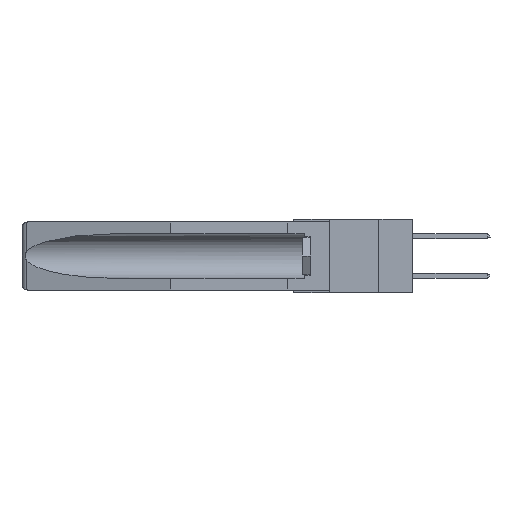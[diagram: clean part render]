
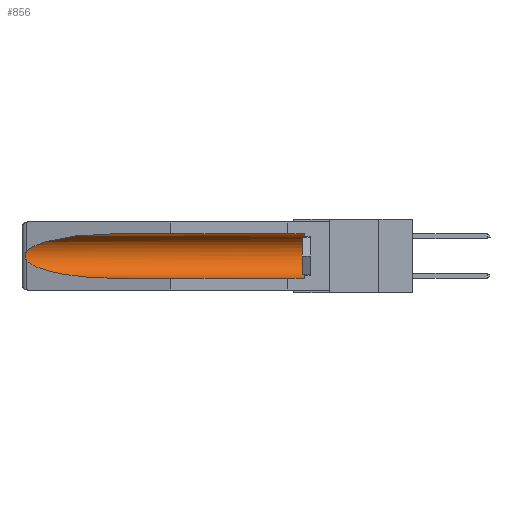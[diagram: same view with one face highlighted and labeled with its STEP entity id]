
A CAD part, left-side view. The second image highlights one B-rep face of the part: STEP entity #856.
In plain terms, the highlighted cylindrical face has radius 2.857 mm (diameter 5.715 mm), a partial arc.
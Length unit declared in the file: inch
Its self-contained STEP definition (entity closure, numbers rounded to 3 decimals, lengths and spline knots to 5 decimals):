
#4 = CARTESIAN_POINT ( 'NONE',  ( 0.26655, 1.53094, -0.18657 ) ) ;
#178 = DIRECTION ( 'NONE',  ( 0., 0., 1. ) ) ;
#856 = ADVANCED_FACE ( 'NONE', ( #16319 ), #3533, .F. ) ;
#969 = VECTOR ( 'NONE', #8975, 39.37008 ) ;
#1082 = ORIENTED_EDGE ( 'NONE', *, *, #8645, .T. ) ;
#1459 = EDGE_CURVE ( 'NONE', #2315, #2692, #11492, .T. ) ;
#2315 = VERTEX_POINT ( 'NONE', #5352 ) ;
#2692 = VERTEX_POINT ( 'NONE', #3282 ) ;
#3206 = ORIENTED_EDGE ( 'NONE', *, *, #9917, .T. ) ;
#3261 = EDGE_CURVE ( 'NONE', #19137, #19927, #17291, .T. ) ;
#3282 = CARTESIAN_POINT ( 'NONE',  ( 0.26537, 1.52718, -0.14972 ) ) ;
#3533 = CYLINDRICAL_SURFACE ( 'NONE', #19335, 0.1125 ) ;
#3579 = VERTEX_POINT ( 'NONE', #5438 ) ;
#3712 = DIRECTION ( 'NONE',  ( 0., 1., 0. ) ) ;
#3803 = CARTESIAN_POINT ( 'NONE',  ( 0.155, 1.07973, -0.284 ) ) ;
#4397 = CARTESIAN_POINT ( 'NONE',  ( 0.26654, 1.53092, -0.15636 ) ) ;
#4469 = EDGE_LOOP ( 'NONE', ( #11773, #3206, #8461, #10026, #18806, #1082 ) ) ;
#5352 = CARTESIAN_POINT ( 'NONE',  ( 0.155, 1.07973, -0.059 ) ) ;
#5438 = CARTESIAN_POINT ( 'NONE',  ( 0.155, 0.126, -0.284 ) ) ;
#5480 = CARTESIAN_POINT ( 'NONE',  ( 0.26537, 1.52718, -0.19328 ) ) ;
#6996 = CARTESIAN_POINT ( 'NONE',  ( 0.25451, 1.48313, -0.24835 ) ) ;
#7425 = CARTESIAN_POINT ( 'NONE',  ( 0.26537, 1.52718, -0.14972 ) ) ;
#7823 = CARTESIAN_POINT ( 'NONE',  ( 0.2675, 1.53308, -0.17534 ) ) ;
#8456 = CARTESIAN_POINT ( 'NONE',  ( 0.21114, 1.30732, -0.059 ) ) ;
#8461 = ORIENTED_EDGE ( 'NONE', *, *, #3261, .T. ) ;
#8645 = EDGE_CURVE ( 'NONE', #19172, #2315, #10836, .T. ) ;
#8659 = CARTESIAN_POINT ( 'NONE',  ( 0.26537, 1.52718, -0.14972 ) ) ;
#8975 = DIRECTION ( 'NONE',  ( 0., 1., 0. ) ) ;
#9210 = EDGE_CURVE ( 'NONE', #3579, #19172, #12037, .T. ) ;
#9917 = EDGE_CURVE ( 'NONE', #2692, #19137, #11753, .T. ) ;
#10026 = ORIENTED_EDGE ( 'NONE', *, *, #10913, .F. ) ;
#10836 = LINE ( 'NONE', #18160, #969 ) ;
#10913 = EDGE_CURVE ( 'NONE', #3579, #19927, #12956, .T. ) ;
#10934 = CARTESIAN_POINT ( 'NONE',  ( 0.26537, 1.52718, -0.19328 ) ) ;
#11492 =( BOUNDED_CURVE ( )  B_SPLINE_CURVE ( 3, ( #11708, #8456, #14905, #8659 ),
 .UNSPECIFIED., .F., .F. ) 
 B_SPLINE_CURVE_WITH_KNOTS ( ( 4, 4 ),
 ( 4.71239, 6.08839 ),
 .UNSPECIFIED. ) 
 CURVE ( )  GEOMETRIC_REPRESENTATION_ITEM ( )  RATIONAL_B_SPLINE_CURVE ( ( 1., 0.848, 0.848, 1. ) ) 
 REPRESENTATION_ITEM ( '' )  );
#11635 = CARTESIAN_POINT ( 'NONE',  ( 0.155, -0.30754, -0.1715 ) ) ;
#11708 = CARTESIAN_POINT ( 'NONE',  ( 0.155, 1.07973, -0.059 ) ) ;
#11753 = B_SPLINE_CURVE_WITH_KNOTS ( 'NONE', 3,
 ( #7425, #12176, #4397, #17113, #20305, #7823, #12513, #4, #15643, #10934 ),
 .UNSPECIFIED., .F., .F.,
 ( 4, 2, 2, 2, 4 ),
 ( 0., 0.00029, 0.00058, 0.00087, 0.00117 ),
 .UNSPECIFIED. ) ;
#11773 = ORIENTED_EDGE ( 'NONE', *, *, #1459, .T. ) ;
#12037 = CIRCLE ( 'NONE', #13025, 0.1125 ) ;
#12176 = CARTESIAN_POINT ( 'NONE',  ( 0.26597, 1.52961, -0.15275 ) ) ;
#12513 = CARTESIAN_POINT ( 'NONE',  ( 0.2673, 1.53269, -0.17917 ) ) ;
#12759 = CARTESIAN_POINT ( 'NONE',  ( 0.155, 0.126, -0.1715 ) ) ;
#12956 = LINE ( 'NONE', #17852, #18828 ) ;
#13025 = AXIS2_PLACEMENT_3D ( 'NONE', #12759, #17231, #178 ) ;
#14693 = DIRECTION ( 'NONE',  ( 0., 0., 1. ) ) ;
#14905 = CARTESIAN_POINT ( 'NONE',  ( 0.25451, 1.48313, -0.09465 ) ) ;
#15643 = CARTESIAN_POINT ( 'NONE',  ( 0.26597, 1.5296, -0.19026 ) ) ;
#16319 = FACE_OUTER_BOUND ( 'NONE', #4469, .T. ) ;
#16401 = CARTESIAN_POINT ( 'NONE',  ( 0.26537, 1.52718, -0.19328 ) ) ;
#17113 = CARTESIAN_POINT ( 'NONE',  ( 0.2673, 1.5327, -0.16383 ) ) ;
#17231 = DIRECTION ( 'NONE',  ( 0., -1., 0. ) ) ;
#17291 =( BOUNDED_CURVE ( )  B_SPLINE_CURVE ( 3, ( #16401, #6996, #17998, #19877 ),
 .UNSPECIFIED., .F., .T. ) 
 B_SPLINE_CURVE_WITH_KNOTS ( ( 4, 4 ),
 ( 0.1948, 1.5708 ),
 .UNSPECIFIED. ) 
 CURVE ( )  GEOMETRIC_REPRESENTATION_ITEM ( )  RATIONAL_B_SPLINE_CURVE ( ( 1., 0.848, 0.848, 1. ) ) 
 REPRESENTATION_ITEM ( '' )  );
#17852 = CARTESIAN_POINT ( 'NONE',  ( 0.155, -0.30754, -0.284 ) ) ;
#17998 = CARTESIAN_POINT ( 'NONE',  ( 0.21114, 1.30732, -0.284 ) ) ;
#18160 = CARTESIAN_POINT ( 'NONE',  ( 0.155, -0.30754, -0.059 ) ) ;
#18806 = ORIENTED_EDGE ( 'NONE', *, *, #9210, .T. ) ;
#18828 = VECTOR ( 'NONE', #19390, 39.37008 ) ;
#19137 = VERTEX_POINT ( 'NONE', #5480 ) ;
#19172 = VERTEX_POINT ( 'NONE', #19439 ) ;
#19335 = AXIS2_PLACEMENT_3D ( 'NONE', #11635, #3712, #14693 ) ;
#19390 = DIRECTION ( 'NONE',  ( 0., 1., 0. ) ) ;
#19439 = CARTESIAN_POINT ( 'NONE',  ( 0.155, 0.126, -0.059 ) ) ;
#19877 = CARTESIAN_POINT ( 'NONE',  ( 0.155, 1.07973, -0.284 ) ) ;
#19927 = VERTEX_POINT ( 'NONE', #3803 ) ;
#20305 = CARTESIAN_POINT ( 'NONE',  ( 0.2675, 1.53308, -0.16763 ) ) ;
